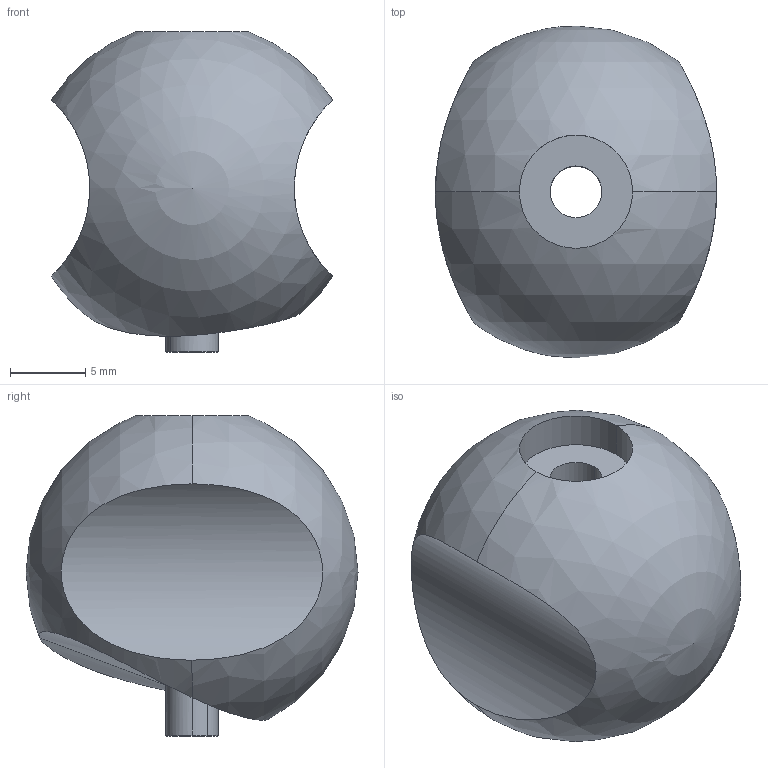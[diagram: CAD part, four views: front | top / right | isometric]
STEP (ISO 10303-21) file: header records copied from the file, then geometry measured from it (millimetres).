
FILE_DESCRIPTION (( 'STEP AP214' ), '1' );
FILE_NAME ('knob2.STEP', '2014-04-06T05:16:08', ( 'eric' ), ( '' ), 'SwSTEP 2.0', 'SolidWorks 2012', '' );
FILE_SCHEMA (( 'AUTOMOTIVE_DESIGN' ));
Length unit declared in the file: millimetre
Products named in the file (1): knob2
Bounding box: 18.64 x 22 x 21.21 mm (x, y, z)
Volume: 4177.1 mm3; surface area: 1737.1 mm2
Topology: 1 solids, 1 shells, 15 faces, 41 edges, 26 vertices
Faces by surface type: cylinder 8, sphere 4, cone 2, plane 1
Entity records: 758 total; most frequent: CARTESIAN_POINT 378, DIRECTION 75, ORIENTED_EDGE 70, EDGE_CURVE 35, AXIS2_PLACEMENT_3D 34, VERTEX_POINT 22, CIRCLE 18, EDGE_LOOP 17
